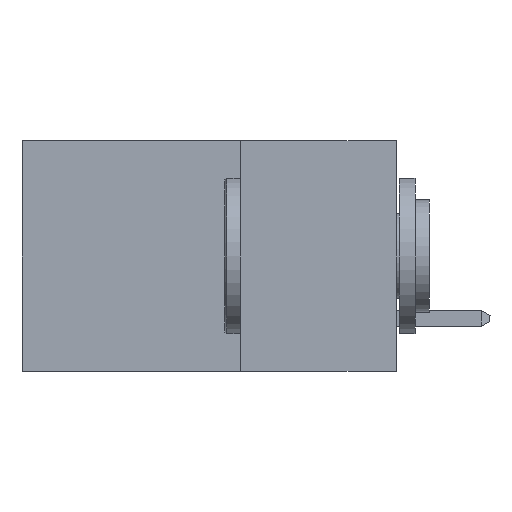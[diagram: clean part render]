
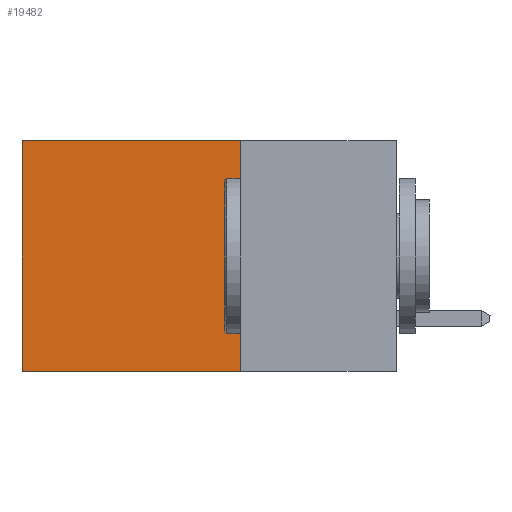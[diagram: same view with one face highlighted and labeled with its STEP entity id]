
A CAD part, left-side view. The second image highlights one B-rep face of the part: STEP entity #19482.
In plain terms, the highlighted planar face has unit normal (-1, 0, 0).
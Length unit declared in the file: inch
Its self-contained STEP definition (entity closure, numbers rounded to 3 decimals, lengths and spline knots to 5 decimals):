
#2188 = CARTESIAN_POINT ( 'NONE',  ( 0.2615, 0.25, 0. ) ) ;
#2305 = ORIENTED_EDGE ( 'NONE', *, *, #14558, .T. ) ;
#3293 = CARTESIAN_POINT ( 'NONE',  ( 0.2615, 0.6, -0.37 ) ) ;
#3378 = DIRECTION ( 'NONE',  ( 0., 1., 0. ) ) ;
#3455 = CARTESIAN_POINT ( 'NONE',  ( 0.2615, 0.25, -0.37 ) ) ;
#4847 = LINE ( 'NONE', #8830, #9208 ) ;
#5222 = VERTEX_POINT ( 'NONE', #3293 ) ;
#5761 = CARTESIAN_POINT ( 'NONE',  ( 0.2615, 0.25, -0.37 ) ) ;
#6400 = VECTOR ( 'NONE', #3378, 39.37008 ) ;
#7710 = CARTESIAN_POINT ( 'NONE',  ( 0.2615, 0.6, 0. ) ) ;
#8754 = FACE_OUTER_BOUND ( 'NONE', #21540, .T. ) ;
#8830 = CARTESIAN_POINT ( 'NONE',  ( 0.2615, 0.6, -0.37 ) ) ;
#9208 = VECTOR ( 'NONE', #22907, 39.37008 ) ;
#9480 = DIRECTION ( 'NONE',  ( 0., 0., -1. ) ) ;
#11339 = LINE ( 'NONE', #3455, #6400 ) ;
#12305 = AXIS2_PLACEMENT_3D ( 'NONE', #5761, #20077, #9480 ) ;
#13069 = DIRECTION ( 'NONE',  ( 0., 0., -1. ) ) ;
#13227 = LINE ( 'NONE', #18239, #16225 ) ;
#14558 = EDGE_CURVE ( 'NONE', #20683, #18275, #19624, .T. ) ;
#14953 = VECTOR ( 'NONE', #16353, 39.37008 ) ;
#15758 = EDGE_CURVE ( 'NONE', #20356, #5222, #11339, .T. ) ;
#16225 = VECTOR ( 'NONE', #13069, 39.37008 ) ;
#16353 = DIRECTION ( 'NONE',  ( 0., 1., 0. ) ) ;
#16375 = CARTESIAN_POINT ( 'NONE',  ( 0.2615, 0.25, 0. ) ) ;
#16535 = PLANE ( 'NONE',  #12305 ) ;
#18239 = CARTESIAN_POINT ( 'NONE',  ( 0.2615, 0.25, -0.37 ) ) ;
#18275 = VERTEX_POINT ( 'NONE', #7710 ) ;
#18376 = ORIENTED_EDGE ( 'NONE', *, *, #20014, .F. ) ;
#19482 = ADVANCED_FACE ( 'NONE', ( #8754 ), #16535, .F. ) ;
#19624 = LINE ( 'NONE', #16375, #14953 ) ;
#20014 = EDGE_CURVE ( 'NONE', #20683, #20356, #13227, .T. ) ;
#20077 = DIRECTION ( 'NONE',  ( 1., 0., 0. ) ) ;
#20356 = VERTEX_POINT ( 'NONE', #22610 ) ;
#20683 = VERTEX_POINT ( 'NONE', #2188 ) ;
#20992 = ORIENTED_EDGE ( 'NONE', *, *, #21774, .T. ) ;
#21540 = EDGE_LOOP ( 'NONE', ( #20992, #22435, #18376, #2305 ) ) ;
#21774 = EDGE_CURVE ( 'NONE', #18275, #5222, #4847, .T. ) ;
#22435 = ORIENTED_EDGE ( 'NONE', *, *, #15758, .F. ) ;
#22610 = CARTESIAN_POINT ( 'NONE',  ( 0.2615, 0.25, -0.37 ) ) ;
#22907 = DIRECTION ( 'NONE',  ( 0., 0., -1. ) ) ;
